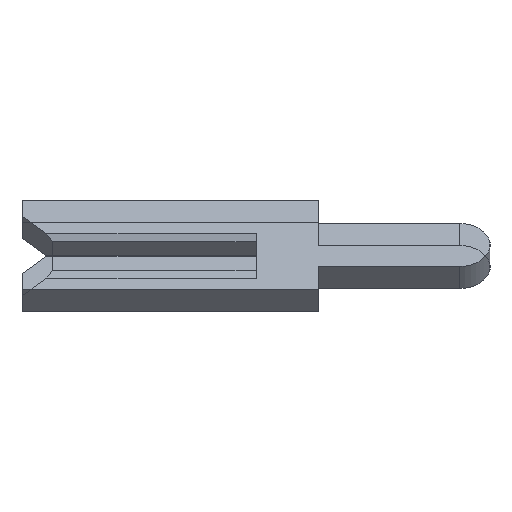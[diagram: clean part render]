
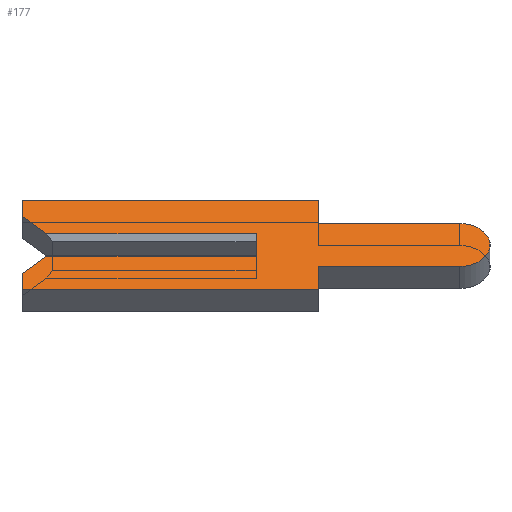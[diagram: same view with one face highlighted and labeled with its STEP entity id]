
A CAD part, left-side view. The second image highlights one B-rep face of the part: STEP entity #177.
In plain terms, the highlighted face is planar.
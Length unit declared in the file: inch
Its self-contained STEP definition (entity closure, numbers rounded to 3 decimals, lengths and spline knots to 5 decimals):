
#54 = EDGE_LOOP ( 'NONE', ( #1777, #681, #1811, #848, #824, #427, #1418, #769, #2293, #258, #1978, #1895, #285, #2059 ) ) ;
#64 = EDGE_CURVE ( 'NONE', #1730, #1945, #737, .T. ) ;
#83 = LINE ( 'NONE', #1231, #1759 ) ;
#168 = DIRECTION ( 'NONE',  ( 0., -1., 0. ) ) ;
#174 = CARTESIAN_POINT ( 'NONE',  ( -0.01, -0.04, -0.04 ) ) ;
#176 = EDGE_CURVE ( 'NONE', #901, #2141, #333, .T. ) ;
#177 = ADVANCED_FACE ( 'NONE', ( #1394 ), #1151, .F. ) ;
#202 = CARTESIAN_POINT ( 'NONE',  ( -0.01, 0.15, -0.04 ) ) ;
#225 = DIRECTION ( 'NONE',  ( 1., 0., 0. ) ) ;
#234 = CARTESIAN_POINT ( 'NONE',  ( -0.01, -0.1305, 0. ) ) ;
#249 = EDGE_CURVE ( 'NONE', #1192, #1831, #1069, .T. ) ;
#258 = ORIENTED_EDGE ( 'NONE', *, *, #937, .F. ) ;
#284 = CARTESIAN_POINT ( 'NONE',  ( -0.01, -0.1305, 0.0195 ) ) ;
#285 = ORIENTED_EDGE ( 'NONE', *, *, #1526, .F. ) ;
#307 = VECTOR ( 'NONE', #829, 39.37008 ) ;
#310 = LINE ( 'NONE', #1598, #1703 ) ;
#314 = DIRECTION ( 'NONE',  ( 0., 0., 1. ) ) ;
#315 = LINE ( 'NONE', #1398, #685 ) ;
#333 = CIRCLE ( 'NONE', #373, 0.0195 ) ;
#339 = VERTEX_POINT ( 'NONE', #2203 ) ;
#373 = AXIS2_PLACEMENT_3D ( 'NONE', #2233, #225, #1692 ) ;
#375 = LINE ( 'NONE', #1566, #2235 ) ;
#407 = LINE ( 'NONE', #1007, #2287 ) ;
#427 = ORIENTED_EDGE ( 'NONE', *, *, #64, .F. ) ;
#442 = DIRECTION ( 'NONE',  ( 0., 0., -1. ) ) ;
#535 = CARTESIAN_POINT ( 'NONE',  ( -0.01, -0.04, -0.04 ) ) ;
#541 = VERTEX_POINT ( 'NONE', #1544 ) ;
#582 = EDGE_CURVE ( 'NONE', #1831, #541, #1015, .T. ) ;
#595 = VECTOR ( 'NONE', #2020, 39.37008 ) ;
#614 = AXIS2_PLACEMENT_3D ( 'NONE', #234, #1136, #442 ) ;
#652 = VECTOR ( 'NONE', #1377, 39.37008 ) ;
#662 = CARTESIAN_POINT ( 'NONE',  ( -0.01, -0.04, 0.04 ) ) ;
#670 = CARTESIAN_POINT ( 'NONE',  ( -0.01, 0.1305, -0.0065 ) ) ;
#681 = ORIENTED_EDGE ( 'NONE', *, *, #582, .F. ) ;
#685 = VECTOR ( 'NONE', #906, 39.37008 ) ;
#715 = DIRECTION ( 'NONE',  ( 0., 0., -1. ) ) ;
#719 = EDGE_CURVE ( 'NONE', #1999, #1071, #1857, .T. ) ;
#737 = LINE ( 'NONE', #202, #1189 ) ;
#769 = ORIENTED_EDGE ( 'NONE', *, *, #1804, .F. ) ;
#813 = CARTESIAN_POINT ( 'NONE',  ( -0.01, 0.15, 0.04 ) ) ;
#824 = ORIENTED_EDGE ( 'NONE', *, *, #1262, .F. ) ;
#826 = EDGE_CURVE ( 'NONE', #1071, #1364, #407, .T. ) ;
#829 = DIRECTION ( 'NONE',  ( 0., 0., 1. ) ) ;
#848 = ORIENTED_EDGE ( 'NONE', *, *, #1019, .F. ) ;
#879 = DIRECTION ( 'NONE',  ( 0., 1., 0. ) ) ;
#901 = VERTEX_POINT ( 'NONE', #284 ) ;
#906 = DIRECTION ( 'NONE',  ( 0., 0., 1. ) ) ;
#914 = CARTESIAN_POINT ( 'NONE',  ( -0.01, -0.1305, -0.0195 ) ) ;
#925 = EDGE_CURVE ( 'NONE', #1916, #2002, #375, .T. ) ;
#932 = CARTESIAN_POINT ( 'NONE',  ( -0.01, 0.134, 0.01 ) ) ;
#937 = EDGE_CURVE ( 'NONE', #1364, #901, #1135, .T. ) ;
#995 = CARTESIAN_POINT ( 'NONE',  ( -0.01, 0., 0.0065 ) ) ;
#1007 = CARTESIAN_POINT ( 'NONE',  ( -0.01, -0.04, 0.04 ) ) ;
#1015 = LINE ( 'NONE', #995, #307 ) ;
#1019 = EDGE_CURVE ( 'NONE', #1834, #1192, #1280, .T. ) ;
#1069 = LINE ( 'NONE', #1676, #595 ) ;
#1071 = VERTEX_POINT ( 'NONE', #662 ) ;
#1087 = DIRECTION ( 'NONE',  ( 0., 1., 0. ) ) ;
#1119 = CARTESIAN_POINT ( 'NONE',  ( -0.01, 0., -0.01 ) ) ;
#1134 = CARTESIAN_POINT ( 'NONE',  ( -0.01, 0.15, 0.04 ) ) ;
#1135 = LINE ( 'NONE', #1716, #2118 ) ;
#1136 = DIRECTION ( 'NONE',  ( 1., 0., 0. ) ) ;
#1151 = PLANE ( 'NONE',  #614 ) ;
#1189 = VECTOR ( 'NONE', #1087, 39.37008 ) ;
#1192 = VERTEX_POINT ( 'NONE', #1407 ) ;
#1231 = CARTESIAN_POINT ( 'NONE',  ( -0.01, 0.15, -0.026 ) ) ;
#1262 = EDGE_CURVE ( 'NONE', #1945, #1834, #83, .T. ) ;
#1280 = LINE ( 'NONE', #670, #1921 ) ;
#1314 = CARTESIAN_POINT ( 'NONE',  ( -0.01, 0.15, -0.04 ) ) ;
#1364 = VERTEX_POINT ( 'NONE', #2108 ) ;
#1373 = DIRECTION ( 'NONE',  ( 0., 0., -1. ) ) ;
#1377 = DIRECTION ( 'NONE',  ( 0., -1., 0. ) ) ;
#1394 = FACE_OUTER_BOUND ( 'NONE', #54, .T. ) ;
#1398 = CARTESIAN_POINT ( 'NONE',  ( -0.01, 0.15, 0.026 ) ) ;
#1407 = CARTESIAN_POINT ( 'NONE',  ( -0.01, 0.134, -0.01 ) ) ;
#1418 = ORIENTED_EDGE ( 'NONE', *, *, #1640, .F. ) ;
#1510 = LINE ( 'NONE', #535, #2006 ) ;
#1526 = EDGE_CURVE ( 'NONE', #2002, #1999, #315, .T. ) ;
#1538 = LINE ( 'NONE', #1803, #2147 ) ;
#1544 = CARTESIAN_POINT ( 'NONE',  ( -0.01, 0., 0.01 ) ) ;
#1566 = CARTESIAN_POINT ( 'NONE',  ( -0.01, 0.1305, 0.0065 ) ) ;
#1598 = CARTESIAN_POINT ( 'NONE',  ( -0.01, 0.15, 0.01 ) ) ;
#1640 = EDGE_CURVE ( 'NONE', #339, #1730, #1510, .T. ) ;
#1676 = CARTESIAN_POINT ( 'NONE',  ( -0.01, -0.1305, -0.01 ) ) ;
#1686 = EDGE_CURVE ( 'NONE', #1916, #541, #310, .T. ) ;
#1692 = DIRECTION ( 'NONE',  ( 0., 0., -1. ) ) ;
#1703 = VECTOR ( 'NONE', #168, 39.37008 ) ;
#1711 = DIRECTION ( 'NONE',  ( 0., 0.707, 0.707 ) ) ;
#1716 = CARTESIAN_POINT ( 'NONE',  ( -0.01, -0.04, 0.0195 ) ) ;
#1730 = VERTEX_POINT ( 'NONE', #174 ) ;
#1759 = VECTOR ( 'NONE', #314, 39.37008 ) ;
#1777 = ORIENTED_EDGE ( 'NONE', *, *, #1686, .T. ) ;
#1803 = CARTESIAN_POINT ( 'NONE',  ( -0.01, -0.04, -0.0195 ) ) ;
#1804 = EDGE_CURVE ( 'NONE', #2141, #339, #1538, .T. ) ;
#1811 = ORIENTED_EDGE ( 'NONE', *, *, #249, .F. ) ;
#1831 = VERTEX_POINT ( 'NONE', #1119 ) ;
#1834 = VERTEX_POINT ( 'NONE', #2144 ) ;
#1857 = LINE ( 'NONE', #813, #652 ) ;
#1895 = ORIENTED_EDGE ( 'NONE', *, *, #719, .F. ) ;
#1916 = VERTEX_POINT ( 'NONE', #932 ) ;
#1921 = VECTOR ( 'NONE', #2126, 39.37008 ) ;
#1945 = VERTEX_POINT ( 'NONE', #1314 ) ;
#1978 = ORIENTED_EDGE ( 'NONE', *, *, #826, .F. ) ;
#1999 = VERTEX_POINT ( 'NONE', #1134 ) ;
#2002 = VERTEX_POINT ( 'NONE', #2209 ) ;
#2006 = VECTOR ( 'NONE', #715, 39.37008 ) ;
#2020 = DIRECTION ( 'NONE',  ( 0., -1., 0. ) ) ;
#2059 = ORIENTED_EDGE ( 'NONE', *, *, #925, .F. ) ;
#2068 = DIRECTION ( 'NONE',  ( 0., -1., 0. ) ) ;
#2108 = CARTESIAN_POINT ( 'NONE',  ( -0.01, -0.04, 0.0195 ) ) ;
#2118 = VECTOR ( 'NONE', #2068, 39.37008 ) ;
#2126 = DIRECTION ( 'NONE',  ( 0., -0.707, 0.707 ) ) ;
#2141 = VERTEX_POINT ( 'NONE', #914 ) ;
#2144 = CARTESIAN_POINT ( 'NONE',  ( -0.01, 0.15, -0.026 ) ) ;
#2147 = VECTOR ( 'NONE', #879, 39.37008 ) ;
#2203 = CARTESIAN_POINT ( 'NONE',  ( -0.01, -0.04, -0.0195 ) ) ;
#2209 = CARTESIAN_POINT ( 'NONE',  ( -0.01, 0.15, 0.026 ) ) ;
#2233 = CARTESIAN_POINT ( 'NONE',  ( -0.01, -0.1305, 0. ) ) ;
#2235 = VECTOR ( 'NONE', #1711, 39.37008 ) ;
#2287 = VECTOR ( 'NONE', #1373, 39.37008 ) ;
#2293 = ORIENTED_EDGE ( 'NONE', *, *, #176, .F. ) ;
